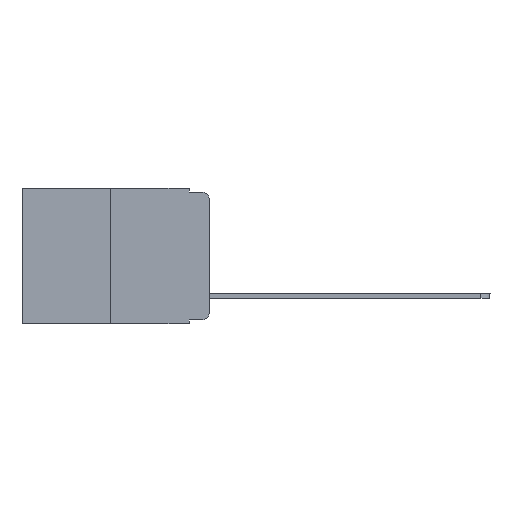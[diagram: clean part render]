
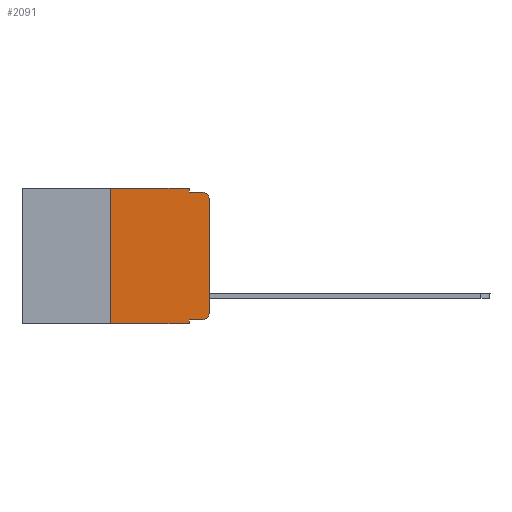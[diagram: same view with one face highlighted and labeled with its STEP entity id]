
A CAD part, left-side view. The second image highlights one B-rep face of the part: STEP entity #2091.
In plain terms, the highlighted planar face has unit normal (-1, 0, 0).
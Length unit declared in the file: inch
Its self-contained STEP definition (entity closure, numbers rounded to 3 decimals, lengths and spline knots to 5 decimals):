
#114 = LINE ( 'NONE', #9439, #6185 ) ;
#186 = DIRECTION ( 'NONE',  ( 0., -1., 0. ) ) ;
#211 = ORIENTED_EDGE ( 'NONE', *, *, #5770, .F. ) ;
#585 = VERTEX_POINT ( 'NONE', #4000 ) ;
#761 = LINE ( 'NONE', #9965, #20476 ) ;
#1984 = LINE ( 'NONE', #11307, #23571 ) ;
#2091 = ADVANCED_FACE ( 'NONE', ( #16971 ), #3756, .F. ) ;
#2131 = EDGE_CURVE ( 'NONE', #13390, #14935, #11975, .T. ) ;
#2692 = VERTEX_POINT ( 'NONE', #2991 ) ;
#2991 = CARTESIAN_POINT ( 'NONE',  ( 0., 0.02, -0.333 ) ) ;
#3756 = PLANE ( 'NONE',  #18017 ) ;
#3802 = DIRECTION ( 'NONE',  ( -1., 0., 0. ) ) ;
#3988 = DIRECTION ( 'NONE',  ( 0., 0., -1. ) ) ;
#4000 = CARTESIAN_POINT ( 'NONE',  ( 0., 0.051, -0.343 ) ) ;
#4117 = DIRECTION ( 'NONE',  ( 1., 0., 0. ) ) ;
#4232 = CARTESIAN_POINT ( 'NONE',  ( 0., 0.473, 0. ) ) ;
#4254 = LINE ( 'NONE', #22780, #8546 ) ;
#4612 = DIRECTION ( 'NONE',  ( 0., -1., 0. ) ) ;
#4651 = VERTEX_POINT ( 'NONE', #17550 ) ;
#5170 = CARTESIAN_POINT ( 'NONE',  ( 0., 0., -0.313 ) ) ;
#5770 = EDGE_CURVE ( 'NONE', #12264, #585, #114, .T. ) ;
#6039 = DIRECTION ( 'NONE',  ( 0., 0., -1. ) ) ;
#6185 = VECTOR ( 'NONE', #3988, 39.37008 ) ;
#6266 = VERTEX_POINT ( 'NONE', #22255 ) ;
#6506 = CARTESIAN_POINT ( 'NONE',  ( 0., 0.051, 0. ) ) ;
#7302 = CARTESIAN_POINT ( 'NONE',  ( 0., 0.02, -0.313 ) ) ;
#7432 = CIRCLE ( 'NONE', #20986, 0.02 ) ;
#7446 = EDGE_CURVE ( 'NONE', #14935, #4651, #22379, .T. ) ;
#7818 = VERTEX_POINT ( 'NONE', #21509 ) ;
#7931 = ORIENTED_EDGE ( 'NONE', *, *, #14049, .T. ) ;
#8546 = VECTOR ( 'NONE', #4612, 39.37008 ) ;
#8580 = DIRECTION ( 'NONE',  ( 0., 0., -1. ) ) ;
#9439 = CARTESIAN_POINT ( 'NONE',  ( 0., 0.051, 0. ) ) ;
#9819 = ORIENTED_EDGE ( 'NONE', *, *, #18386, .F. ) ;
#9965 = CARTESIAN_POINT ( 'NONE',  ( 0., 0.25, 0. ) ) ;
#10679 = VECTOR ( 'NONE', #10833, 39.37008 ) ;
#10833 = DIRECTION ( 'NONE',  ( 0., -1., 0. ) ) ;
#11237 = DIRECTION ( 'NONE',  ( 0., -1., 0. ) ) ;
#11294 = CARTESIAN_POINT ( 'NONE',  ( 0., 0.25, 0. ) ) ;
#11307 = CARTESIAN_POINT ( 'NONE',  ( 0., 0., 0. ) ) ;
#11476 = EDGE_LOOP ( 'NONE', ( #16587, #13546, #12832, #15703, #9819, #17104, #7931, #211, #22978, #12510 ) ) ;
#11949 = EDGE_CURVE ( 'NONE', #12264, #2692, #22959, .T. ) ;
#11973 = EDGE_CURVE ( 'NONE', #6266, #4651, #20361, .T. ) ;
#11975 = LINE ( 'NONE', #6506, #12601 ) ;
#12264 = VERTEX_POINT ( 'NONE', #22930 ) ;
#12510 = ORIENTED_EDGE ( 'NONE', *, *, #19585, .T. ) ;
#12601 = VECTOR ( 'NONE', #8580, 39.37008 ) ;
#12832 = ORIENTED_EDGE ( 'NONE', *, *, #7446, .F. ) ;
#12905 = DIRECTION ( 'NONE',  ( 0., 0., -1. ) ) ;
#13390 = VERTEX_POINT ( 'NONE', #20867 ) ;
#13546 = ORIENTED_EDGE ( 'NONE', *, *, #11973, .T. ) ;
#14049 = EDGE_CURVE ( 'NONE', #7818, #585, #14843, .T. ) ;
#14546 = EDGE_CURVE ( 'NONE', #15634, #6266, #1984, .T. ) ;
#14843 = LINE ( 'NONE', #18964, #16199 ) ;
#14935 = VERTEX_POINT ( 'NONE', #16736 ) ;
#15634 = VERTEX_POINT ( 'NONE', #5170 ) ;
#15703 = ORIENTED_EDGE ( 'NONE', *, *, #2131, .F. ) ;
#16199 = VECTOR ( 'NONE', #186, 39.37008 ) ;
#16587 = ORIENTED_EDGE ( 'NONE', *, *, #14546, .T. ) ;
#16736 = CARTESIAN_POINT ( 'NONE',  ( 0., 0.051, -0.01 ) ) ;
#16971 = FACE_OUTER_BOUND ( 'NONE', #11476, .T. ) ;
#17104 = ORIENTED_EDGE ( 'NONE', *, *, #23338, .F. ) ;
#17550 = CARTESIAN_POINT ( 'NONE',  ( 0., 0.02, -0.01 ) ) ;
#18017 = AXIS2_PLACEMENT_3D ( 'NONE', #4232, #4117, #6039 ) ;
#18111 = DIRECTION ( 'NONE',  ( -1., 0., 0. ) ) ;
#18386 = EDGE_CURVE ( 'NONE', #22387, #13390, #4254, .T. ) ;
#18701 = DIRECTION ( 'NONE',  ( 0., 0., 1. ) ) ;
#18964 = CARTESIAN_POINT ( 'NONE',  ( 0., 0.473, -0.343 ) ) ;
#19076 = DIRECTION ( 'NONE',  ( 0., 0., 1. ) ) ;
#19585 = EDGE_CURVE ( 'NONE', #2692, #15634, #7432, .T. ) ;
#19929 = DIRECTION ( 'NONE',  ( 0., 0., -1. ) ) ;
#19974 = AXIS2_PLACEMENT_3D ( 'NONE', #21744, #18111, #19929 ) ;
#20361 = CIRCLE ( 'NONE', #19974, 0.02 ) ;
#20476 = VECTOR ( 'NONE', #19076, 39.37008 ) ;
#20867 = CARTESIAN_POINT ( 'NONE',  ( 0., 0.051, 0. ) ) ;
#20986 = AXIS2_PLACEMENT_3D ( 'NONE', #7302, #3802, #12905 ) ;
#21142 = CARTESIAN_POINT ( 'NONE',  ( 0., 0.051, -0.333 ) ) ;
#21397 = VECTOR ( 'NONE', #11237, 39.37008 ) ;
#21509 = CARTESIAN_POINT ( 'NONE',  ( 0., 0.25, -0.343 ) ) ;
#21744 = CARTESIAN_POINT ( 'NONE',  ( 0., 0.02, -0.03 ) ) ;
#22255 = CARTESIAN_POINT ( 'NONE',  ( 0., 0., -0.03 ) ) ;
#22379 = LINE ( 'NONE', #22612, #21397 ) ;
#22387 = VERTEX_POINT ( 'NONE', #11294 ) ;
#22612 = CARTESIAN_POINT ( 'NONE',  ( 0., 0.051, -0.01 ) ) ;
#22780 = CARTESIAN_POINT ( 'NONE',  ( 0., 0.473, 0. ) ) ;
#22930 = CARTESIAN_POINT ( 'NONE',  ( 0., 0.051, -0.333 ) ) ;
#22959 = LINE ( 'NONE', #21142, #10679 ) ;
#22978 = ORIENTED_EDGE ( 'NONE', *, *, #11949, .T. ) ;
#23338 = EDGE_CURVE ( 'NONE', #7818, #22387, #761, .T. ) ;
#23571 = VECTOR ( 'NONE', #18701, 39.37008 ) ;
